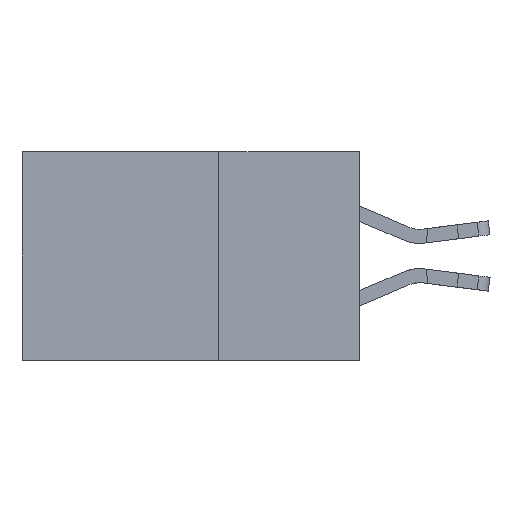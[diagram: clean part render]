
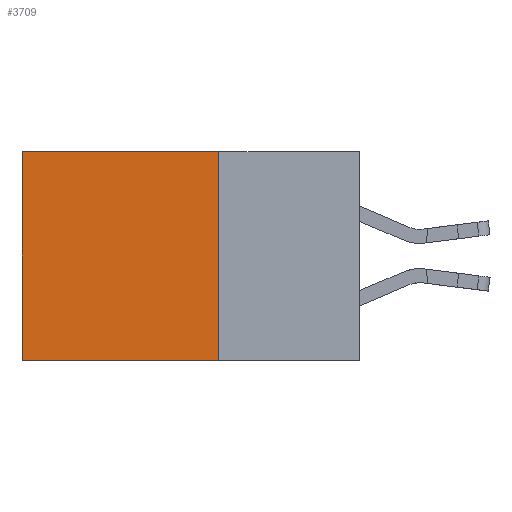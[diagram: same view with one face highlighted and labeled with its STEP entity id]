
A CAD part, left-side view. The second image highlights one B-rep face of the part: STEP entity #3709.
In plain terms, the highlighted planar face has unit normal (-1, 0, 0).
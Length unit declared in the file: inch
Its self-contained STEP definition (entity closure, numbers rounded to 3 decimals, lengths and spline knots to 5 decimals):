
#182 = DIRECTION ( 'NONE',  ( 0., 1., 0. ) ) ;
#268 = ORIENTED_EDGE ( 'NONE', *, *, #14329, .T. ) ;
#1013 = EDGE_CURVE ( 'NONE', #14758, #13530, #7180, .T. ) ;
#1186 = CARTESIAN_POINT ( 'NONE',  ( 0.2875, 0.25, 0. ) ) ;
#1492 = EDGE_LOOP ( 'NONE', ( #17287, #20042, #6753, #268 ) ) ;
#1605 = VECTOR ( 'NONE', #17485, 39.37008 ) ;
#1687 = VERTEX_POINT ( 'NONE', #18560 ) ;
#1955 = VECTOR ( 'NONE', #7651, 39.37008 ) ;
#2763 = LINE ( 'NONE', #20686, #19847 ) ;
#3709 = ADVANCED_FACE ( 'NONE', ( #14477 ), #9624, .F. ) ;
#4433 = CARTESIAN_POINT ( 'NONE',  ( 0.2875, 0.25, 0. ) ) ;
#5186 = CARTESIAN_POINT ( 'NONE',  ( 0.2875, 0.25, -0.37 ) ) ;
#6195 = DIRECTION ( 'NONE',  ( 1., 0., 0. ) ) ;
#6753 = ORIENTED_EDGE ( 'NONE', *, *, #1013, .F. ) ;
#7180 = LINE ( 'NONE', #1186, #1955 ) ;
#7391 = CARTESIAN_POINT ( 'NONE',  ( 0.2875, 0.25, 0. ) ) ;
#7651 = DIRECTION ( 'NONE',  ( 0., 0., -1. ) ) ;
#9624 = PLANE ( 'NONE',  #19965 ) ;
#10308 = CARTESIAN_POINT ( 'NONE',  ( 0.2875, 0.25, 0. ) ) ;
#13530 = VERTEX_POINT ( 'NONE', #5186 ) ;
#13624 = EDGE_CURVE ( 'NONE', #13530, #21896, #2763, .T. ) ;
#13746 = LINE ( 'NONE', #19425, #21594 ) ;
#14329 = EDGE_CURVE ( 'NONE', #14758, #1687, #15844, .T. ) ;
#14438 = EDGE_CURVE ( 'NONE', #1687, #21896, #13746, .T. ) ;
#14477 = FACE_OUTER_BOUND ( 'NONE', #1492, .T. ) ;
#14758 = VERTEX_POINT ( 'NONE', #10308 ) ;
#15844 = LINE ( 'NONE', #7391, #1605 ) ;
#15965 = CARTESIAN_POINT ( 'NONE',  ( 0.2875, 0.6, -0.37 ) ) ;
#17287 = ORIENTED_EDGE ( 'NONE', *, *, #14438, .T. ) ;
#17485 = DIRECTION ( 'NONE',  ( 0., 1., 0. ) ) ;
#17706 = DIRECTION ( 'NONE',  ( 0., 0., -1. ) ) ;
#18053 = DIRECTION ( 'NONE',  ( 0., 0., -1. ) ) ;
#18560 = CARTESIAN_POINT ( 'NONE',  ( 0.2875, 0.6, 0. ) ) ;
#19425 = CARTESIAN_POINT ( 'NONE',  ( 0.2875, 0.6, 0. ) ) ;
#19847 = VECTOR ( 'NONE', #182, 39.37008 ) ;
#19965 = AXIS2_PLACEMENT_3D ( 'NONE', #4433, #6195, #18053 ) ;
#20042 = ORIENTED_EDGE ( 'NONE', *, *, #13624, .F. ) ;
#20686 = CARTESIAN_POINT ( 'NONE',  ( 0.2875, 0.25, -0.37 ) ) ;
#21594 = VECTOR ( 'NONE', #17706, 39.37008 ) ;
#21896 = VERTEX_POINT ( 'NONE', #15965 ) ;
